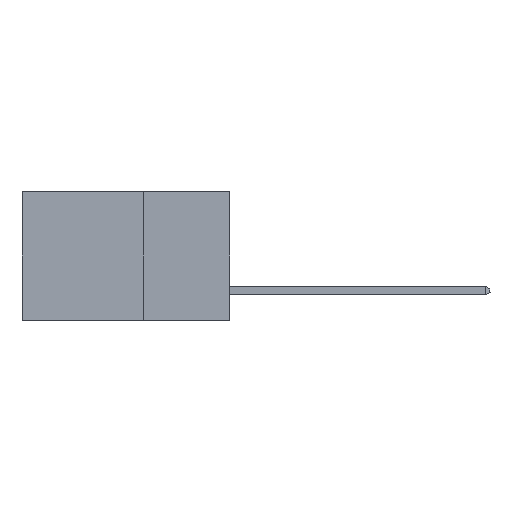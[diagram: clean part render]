
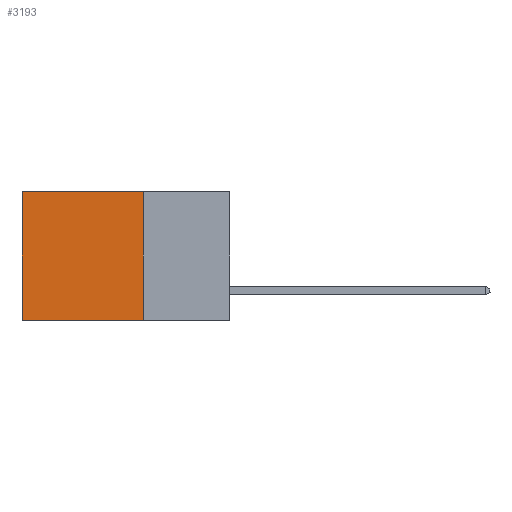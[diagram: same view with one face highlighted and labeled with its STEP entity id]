
A CAD part, left-side view. The second image highlights one B-rep face of the part: STEP entity #3193.
In plain terms, the highlighted planar face has unit normal (-1, 0, 0).
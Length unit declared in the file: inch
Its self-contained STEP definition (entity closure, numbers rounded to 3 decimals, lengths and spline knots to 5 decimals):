
#147 = EDGE_CURVE ( 'NONE', #9594, #2776, #15414, .T. ) ;
#193 = VERTEX_POINT ( 'NONE', #13755 ) ;
#577 = CARTESIAN_POINT ( 'NONE',  ( 0.298, 0.25, -0.37 ) ) ;
#1800 = EDGE_CURVE ( 'NONE', #2776, #10357, #8047, .T. ) ;
#2260 = EDGE_CURVE ( 'NONE', #193, #10357, #2874, .T. ) ;
#2413 = PLANE ( 'NONE',  #12152 ) ;
#2776 = VERTEX_POINT ( 'NONE', #9926 ) ;
#2874 = LINE ( 'NONE', #577, #17957 ) ;
#2928 = CARTESIAN_POINT ( 'NONE',  ( 0.298, 0.6, 0. ) ) ;
#3193 = ADVANCED_FACE ( 'NONE', ( #17665 ), #2413, .F. ) ;
#3382 = CARTESIAN_POINT ( 'NONE',  ( 0.298, 0.25, 0. ) ) ;
#3498 = CARTESIAN_POINT ( 'NONE',  ( 0.298, 0.25, 0. ) ) ;
#4240 = ORIENTED_EDGE ( 'NONE', *, *, #2260, .F. ) ;
#4694 = DIRECTION ( 'NONE',  ( 0., 0., -1. ) ) ;
#6378 = ORIENTED_EDGE ( 'NONE', *, *, #147, .T. ) ;
#6987 = DIRECTION ( 'NONE',  ( 0., 0., -1. ) ) ;
#7484 = VECTOR ( 'NONE', #4694, 39.37008 ) ;
#7626 = CARTESIAN_POINT ( 'NONE',  ( 0.298, 0.6, -0.37 ) ) ;
#8047 = LINE ( 'NONE', #2928, #7484 ) ;
#8511 = DIRECTION ( 'NONE',  ( 0., 1., 0. ) ) ;
#8772 = DIRECTION ( 'NONE',  ( 1., 0., 0. ) ) ;
#9594 = VERTEX_POINT ( 'NONE', #16409 ) ;
#9926 = CARTESIAN_POINT ( 'NONE',  ( 0.298, 0.6, 0. ) ) ;
#10357 = VERTEX_POINT ( 'NONE', #7626 ) ;
#11351 = VECTOR ( 'NONE', #22659, 39.37008 ) ;
#12099 = CARTESIAN_POINT ( 'NONE',  ( 0.298, 0.25, 0. ) ) ;
#12152 = AXIS2_PLACEMENT_3D ( 'NONE', #3498, #8772, #6987 ) ;
#13755 = CARTESIAN_POINT ( 'NONE',  ( 0.298, 0.25, -0.37 ) ) ;
#14120 = EDGE_LOOP ( 'NONE', ( #19397, #4240, #18950, #6378 ) ) ;
#14211 = EDGE_CURVE ( 'NONE', #9594, #193, #16055, .T. ) ;
#14433 = DIRECTION ( 'NONE',  ( 0., 1., 0. ) ) ;
#15414 = LINE ( 'NONE', #12099, #18682 ) ;
#16055 = LINE ( 'NONE', #3382, #11351 ) ;
#16409 = CARTESIAN_POINT ( 'NONE',  ( 0.298, 0.25, 0. ) ) ;
#17665 = FACE_OUTER_BOUND ( 'NONE', #14120, .T. ) ;
#17957 = VECTOR ( 'NONE', #14433, 39.37008 ) ;
#18682 = VECTOR ( 'NONE', #8511, 39.37008 ) ;
#18950 = ORIENTED_EDGE ( 'NONE', *, *, #14211, .F. ) ;
#19397 = ORIENTED_EDGE ( 'NONE', *, *, #1800, .T. ) ;
#22659 = DIRECTION ( 'NONE',  ( 0., 0., -1. ) ) ;
